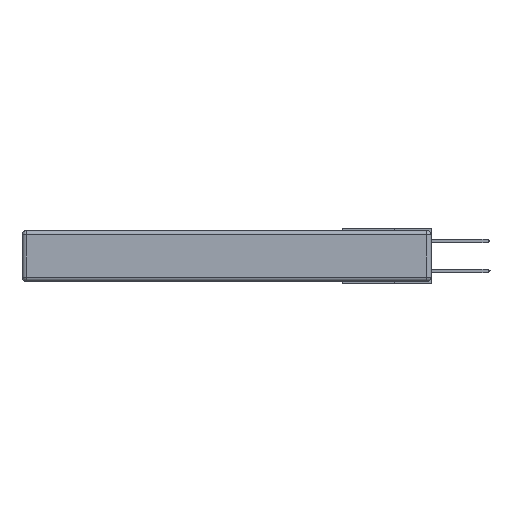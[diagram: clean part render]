
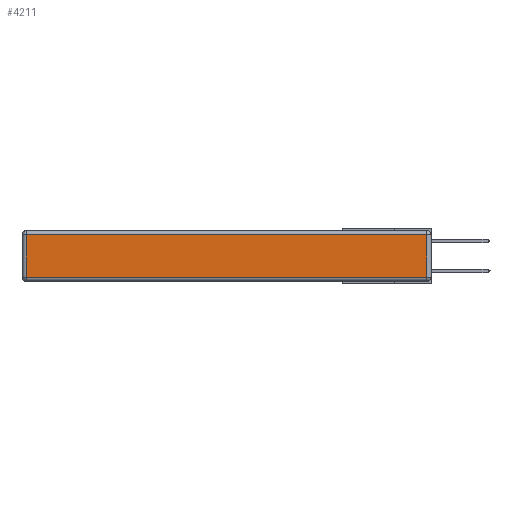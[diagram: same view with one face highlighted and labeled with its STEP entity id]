
A CAD part, left-side view. The second image highlights one B-rep face of the part: STEP entity #4211.
In plain terms, the highlighted planar face has unit normal (-1, 0, 0).
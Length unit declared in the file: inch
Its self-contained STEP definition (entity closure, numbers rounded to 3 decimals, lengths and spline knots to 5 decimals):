
#491 = VECTOR ( 'NONE', #2685, 39.37008 ) ;
#551 = CARTESIAN_POINT ( 'NONE',  ( 0., 2.72, -0.313 ) ) ;
#1062 = VERTEX_POINT ( 'NONE', #6387 ) ;
#1365 = VERTEX_POINT ( 'NONE', #13965 ) ;
#1521 = VECTOR ( 'NONE', #4907, 39.37008 ) ;
#1773 = EDGE_CURVE ( 'NONE', #16012, #11681, #7023, .T. ) ;
#2326 = CARTESIAN_POINT ( 'NONE',  ( 0., 0., -0.343 ) ) ;
#2685 = DIRECTION ( 'NONE',  ( 0., 1., 0. ) ) ;
#3052 = ORIENTED_EDGE ( 'NONE', *, *, #7634, .T. ) ;
#3584 = CARTESIAN_POINT ( 'NONE',  ( 0., 0.03, -0.343 ) ) ;
#4211 = ADVANCED_FACE ( 'NONE', ( #8863 ), #7881, .T. ) ;
#4484 = EDGE_LOOP ( 'NONE', ( #16400, #6723, #3052, #14324 ) ) ;
#4907 = DIRECTION ( 'NONE',  ( 0., 0., 1. ) ) ;
#5554 = DIRECTION ( 'NONE',  ( 0., 0., -1. ) ) ;
#6159 = CARTESIAN_POINT ( 'NONE',  ( 0., 0.03, -0.313 ) ) ;
#6387 = CARTESIAN_POINT ( 'NONE',  ( 0., 0.03, -0.03 ) ) ;
#6723 = ORIENTED_EDGE ( 'NONE', *, *, #11219, .T. ) ;
#7023 = LINE ( 'NONE', #10693, #8742 ) ;
#7047 = CARTESIAN_POINT ( 'NONE',  ( 0., 2.72, -0.343 ) ) ;
#7634 = EDGE_CURVE ( 'NONE', #1062, #1365, #12172, .T. ) ;
#7881 = PLANE ( 'NONE',  #9250 ) ;
#8384 = VECTOR ( 'NONE', #5554, 39.37008 ) ;
#8742 = VECTOR ( 'NONE', #10639, 39.37008 ) ;
#8863 = FACE_OUTER_BOUND ( 'NONE', #4484, .T. ) ;
#9219 = DIRECTION ( 'NONE',  ( -1., 0., 0. ) ) ;
#9250 = AXIS2_PLACEMENT_3D ( 'NONE', #2326, #9219, #14766 ) ;
#10570 = LINE ( 'NONE', #7047, #8384 ) ;
#10617 = LINE ( 'NONE', #3584, #1521 ) ;
#10639 = DIRECTION ( 'NONE',  ( 0., -1., 0. ) ) ;
#10693 = CARTESIAN_POINT ( 'NONE',  ( 0., 0., -0.313 ) ) ;
#11219 = EDGE_CURVE ( 'NONE', #11681, #1062, #10617, .T. ) ;
#11681 = VERTEX_POINT ( 'NONE', #6159 ) ;
#12172 = LINE ( 'NONE', #16556, #491 ) ;
#13299 = EDGE_CURVE ( 'NONE', #1365, #16012, #10570, .T. ) ;
#13965 = CARTESIAN_POINT ( 'NONE',  ( 0., 2.72, -0.03 ) ) ;
#14324 = ORIENTED_EDGE ( 'NONE', *, *, #13299, .T. ) ;
#14766 = DIRECTION ( 'NONE',  ( 0., 0., 1. ) ) ;
#16012 = VERTEX_POINT ( 'NONE', #551 ) ;
#16400 = ORIENTED_EDGE ( 'NONE', *, *, #1773, .T. ) ;
#16556 = CARTESIAN_POINT ( 'NONE',  ( 0., 2.75, -0.03 ) ) ;
